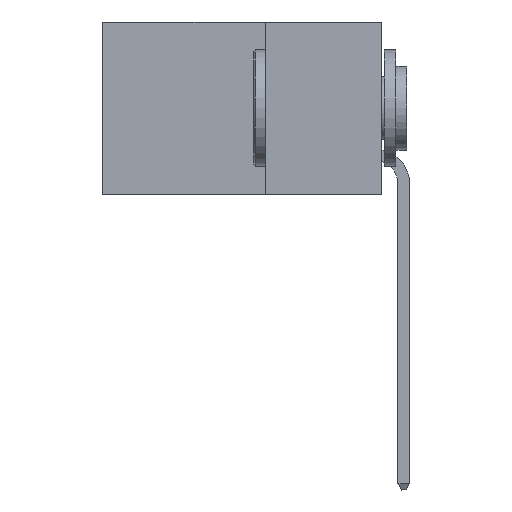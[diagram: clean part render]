
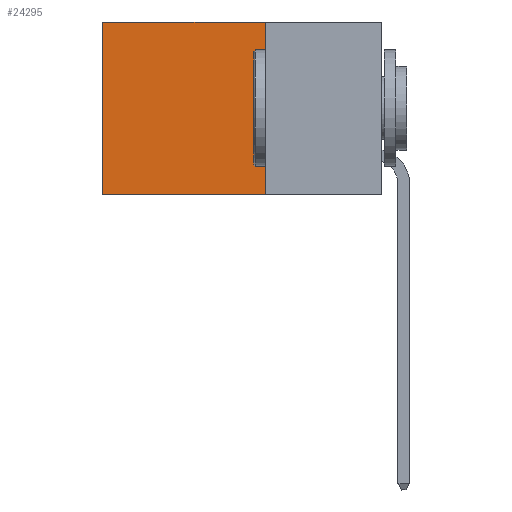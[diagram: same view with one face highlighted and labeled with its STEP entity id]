
A CAD part, left-side view. The second image highlights one B-rep face of the part: STEP entity #24295.
In plain terms, the highlighted planar face has unit normal (-1, 0, 0).
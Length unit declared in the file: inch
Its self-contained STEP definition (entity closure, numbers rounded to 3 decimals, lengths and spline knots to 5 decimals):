
#640 = VECTOR ( 'NONE', #24921, 39.37008 ) ;
#1220 = ORIENTED_EDGE ( 'NONE', *, *, #36945, .T. ) ;
#2154 = ORIENTED_EDGE ( 'NONE', *, *, #15328, .F. ) ;
#3322 = CARTESIAN_POINT ( 'NONE',  ( 0.2875, 0.25, 0. ) ) ;
#3773 = EDGE_CURVE ( 'NONE', #14905, #37500, #41412, .T. ) ;
#4813 = VERTEX_POINT ( 'NONE', #34325 ) ;
#6252 = PLANE ( 'NONE',  #16543 ) ;
#6552 = DIRECTION ( 'NONE',  ( 0., 0., -1. ) ) ;
#9830 = DIRECTION ( 'NONE',  ( 1., 0., 0. ) ) ;
#10416 = CARTESIAN_POINT ( 'NONE',  ( 0.2875, 0.6, 0. ) ) ;
#11249 = VECTOR ( 'NONE', #12447, 39.37008 ) ;
#12447 = DIRECTION ( 'NONE',  ( 0., 1., 0. ) ) ;
#14905 = VERTEX_POINT ( 'NONE', #18270 ) ;
#15328 = EDGE_CURVE ( 'NONE', #4813, #35695, #26948, .T. ) ;
#16543 = AXIS2_PLACEMENT_3D ( 'NONE', #3322, #9830, #39290 ) ;
#17567 = VECTOR ( 'NONE', #6552, 39.37008 ) ;
#18270 = CARTESIAN_POINT ( 'NONE',  ( 0.2875, 0.6, 0. ) ) ;
#18352 = ORIENTED_EDGE ( 'NONE', *, *, #41479, .F. ) ;
#19621 = EDGE_LOOP ( 'NONE', ( #35556, #18352, #2154, #1220 ) ) ;
#19980 = LINE ( 'NONE', #22254, #11249 ) ;
#21558 = CARTESIAN_POINT ( 'NONE',  ( 0.2875, 0.25, 0. ) ) ;
#22254 = CARTESIAN_POINT ( 'NONE',  ( 0.2875, 0.25, -0.37 ) ) ;
#24295 = ADVANCED_FACE ( 'NONE', ( #41795 ), #6252, .F. ) ;
#24921 = DIRECTION ( 'NONE',  ( 0., 1., 0. ) ) ;
#26948 = LINE ( 'NONE', #33710, #28006 ) ;
#28006 = VECTOR ( 'NONE', #33861, 39.37008 ) ;
#30758 = CARTESIAN_POINT ( 'NONE',  ( 0.2875, 0.6, -0.37 ) ) ;
#33710 = CARTESIAN_POINT ( 'NONE',  ( 0.2875, 0.25, 0. ) ) ;
#33861 = DIRECTION ( 'NONE',  ( 0., 0., -1. ) ) ;
#34325 = CARTESIAN_POINT ( 'NONE',  ( 0.2875, 0.25, 0. ) ) ;
#35217 = CARTESIAN_POINT ( 'NONE',  ( 0.2875, 0.25, -0.37 ) ) ;
#35556 = ORIENTED_EDGE ( 'NONE', *, *, #3773, .T. ) ;
#35695 = VERTEX_POINT ( 'NONE', #35217 ) ;
#36945 = EDGE_CURVE ( 'NONE', #4813, #14905, #37875, .T. ) ;
#37500 = VERTEX_POINT ( 'NONE', #30758 ) ;
#37875 = LINE ( 'NONE', #21558, #640 ) ;
#39290 = DIRECTION ( 'NONE',  ( 0., 0., -1. ) ) ;
#41412 = LINE ( 'NONE', #10416, #17567 ) ;
#41479 = EDGE_CURVE ( 'NONE', #35695, #37500, #19980, .T. ) ;
#41795 = FACE_OUTER_BOUND ( 'NONE', #19621, .T. ) ;
